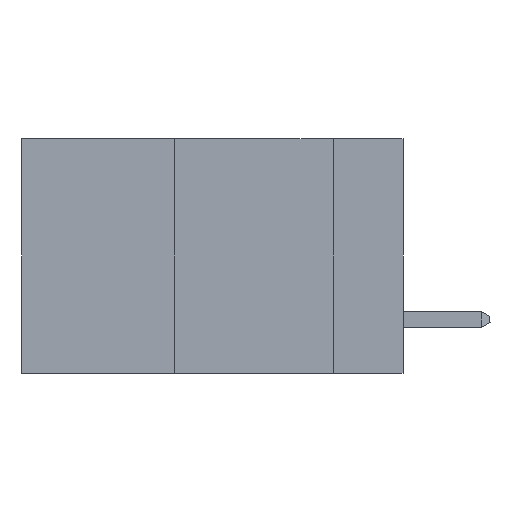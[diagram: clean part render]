
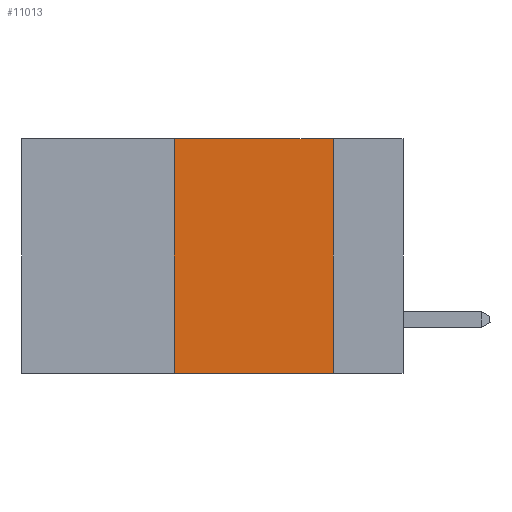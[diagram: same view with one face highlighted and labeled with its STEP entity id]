
A CAD part, left-side view. The second image highlights one B-rep face of the part: STEP entity #11013.
In plain terms, the highlighted planar face has unit normal (-1, 0, 0).
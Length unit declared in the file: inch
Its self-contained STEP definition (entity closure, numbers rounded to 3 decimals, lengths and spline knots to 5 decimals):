
#1932 = VECTOR ( 'NONE', #13872, 39.37008 ) ;
#2092 = CARTESIAN_POINT ( 'NONE',  ( 0., 0.6, 0. ) ) ;
#2176 = EDGE_CURVE ( 'NONE', #18605, #16332, #5479, .T. ) ;
#2676 = VECTOR ( 'NONE', #21996, 39.37008 ) ;
#3249 = CARTESIAN_POINT ( 'NONE',  ( 0., 0.6, -0.37 ) ) ;
#4078 = CARTESIAN_POINT ( 'NONE',  ( 0., 0.11, -0.37 ) ) ;
#4905 = CARTESIAN_POINT ( 'NONE',  ( 0., 0.11, 0. ) ) ;
#5479 = LINE ( 'NONE', #2092, #10367 ) ;
#6184 = DIRECTION ( 'NONE',  ( 0., 0., -1. ) ) ;
#6925 = LINE ( 'NONE', #4905, #1932 ) ;
#7125 = AXIS2_PLACEMENT_3D ( 'NONE', #18576, #16852, #6184 ) ;
#7389 = FACE_OUTER_BOUND ( 'NONE', #18513, .T. ) ;
#7630 = LINE ( 'NONE', #7979, #2676 ) ;
#7979 = CARTESIAN_POINT ( 'NONE',  ( 0., 0.36, 0. ) ) ;
#10204 = VECTOR ( 'NONE', #12418, 39.37008 ) ;
#10367 = VECTOR ( 'NONE', #18249, 39.37008 ) ;
#11013 = ADVANCED_FACE ( 'NONE', ( #7389 ), #11605, .F. ) ;
#11605 = PLANE ( 'NONE',  #7125 ) ;
#12335 = EDGE_CURVE ( 'NONE', #17290, #18605, #7630, .T. ) ;
#12418 = DIRECTION ( 'NONE',  ( 0., -1., 0. ) ) ;
#13872 = DIRECTION ( 'NONE',  ( 0., 0., -1. ) ) ;
#14791 = EDGE_CURVE ( 'NONE', #16332, #15762, #6925, .T. ) ;
#15762 = VERTEX_POINT ( 'NONE', #4078 ) ;
#15920 = ORIENTED_EDGE ( 'NONE', *, *, #12335, .F. ) ;
#16332 = VERTEX_POINT ( 'NONE', #17070 ) ;
#16852 = DIRECTION ( 'NONE',  ( 1., 0., 0. ) ) ;
#17070 = CARTESIAN_POINT ( 'NONE',  ( 0., 0.11, 0. ) ) ;
#17290 = VERTEX_POINT ( 'NONE', #22893 ) ;
#18194 = ORIENTED_EDGE ( 'NONE', *, *, #22540, .T. ) ;
#18249 = DIRECTION ( 'NONE',  ( 0., -1., 0. ) ) ;
#18513 = EDGE_LOOP ( 'NONE', ( #22303, #22637, #15920, #18194 ) ) ;
#18576 = CARTESIAN_POINT ( 'NONE',  ( 0., 0.6, 0. ) ) ;
#18605 = VERTEX_POINT ( 'NONE', #20931 ) ;
#20077 = LINE ( 'NONE', #3249, #10204 ) ;
#20931 = CARTESIAN_POINT ( 'NONE',  ( 0., 0.36, 0. ) ) ;
#21996 = DIRECTION ( 'NONE',  ( 0., 0., 1. ) ) ;
#22303 = ORIENTED_EDGE ( 'NONE', *, *, #14791, .F. ) ;
#22540 = EDGE_CURVE ( 'NONE', #17290, #15762, #20077, .T. ) ;
#22637 = ORIENTED_EDGE ( 'NONE', *, *, #2176, .F. ) ;
#22893 = CARTESIAN_POINT ( 'NONE',  ( 0., 0.36, -0.37 ) ) ;
